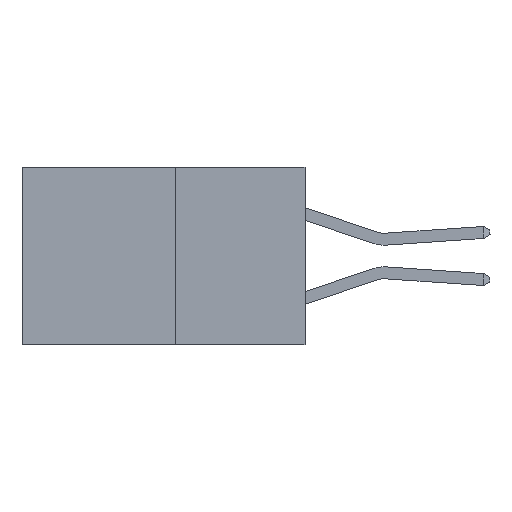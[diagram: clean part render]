
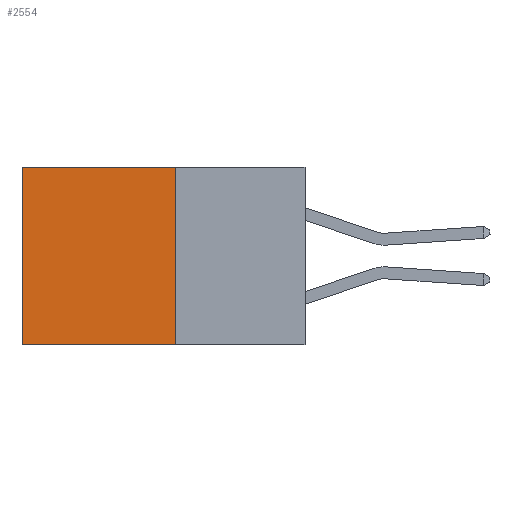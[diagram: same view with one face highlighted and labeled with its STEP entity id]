
A CAD part, left-side view. The second image highlights one B-rep face of the part: STEP entity #2554.
In plain terms, the highlighted planar face has unit normal (-1, 0, 0).
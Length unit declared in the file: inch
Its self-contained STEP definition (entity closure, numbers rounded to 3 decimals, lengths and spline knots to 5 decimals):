
#334 = ORIENTED_EDGE ( 'NONE', *, *, #688, .F. ) ;
#534 = AXIS2_PLACEMENT_3D ( 'NONE', #11192, #17111, #16595 ) ;
#688 = EDGE_CURVE ( 'NONE', #1256, #17459, #8803, .T. ) ;
#799 = ORIENTED_EDGE ( 'NONE', *, *, #17157, .F. ) ;
#933 = DIRECTION ( 'NONE',  ( 0., 1., 0. ) ) ;
#1256 = VERTEX_POINT ( 'NONE', #10063 ) ;
#1376 = EDGE_CURVE ( 'NONE', #4026, #14913, #4610, .T. ) ;
#1718 = ORIENTED_EDGE ( 'NONE', *, *, #1376, .T. ) ;
#2058 = FACE_OUTER_BOUND ( 'NONE', #18214, .T. ) ;
#2374 = CARTESIAN_POINT ( 'NONE',  ( 0.277, 0.59, -0.37 ) ) ;
#2554 = ADVANCED_FACE ( 'NONE', ( #2058 ), #17402, .F. ) ;
#2951 = LINE ( 'NONE', #19134, #11455 ) ;
#4026 = VERTEX_POINT ( 'NONE', #19067 ) ;
#4610 = LINE ( 'NONE', #9505, #8307 ) ;
#4878 = CARTESIAN_POINT ( 'NONE',  ( 0.277, 0.27, -0.37 ) ) ;
#4965 = DIRECTION ( 'NONE',  ( 0., 0., -1. ) ) ;
#6169 = VECTOR ( 'NONE', #14476, 39.37008 ) ;
#6694 = ORIENTED_EDGE ( 'NONE', *, *, #9288, .T. ) ;
#7139 = LINE ( 'NONE', #15082, #6169 ) ;
#8074 = DIRECTION ( 'NONE',  ( 0., 1., 0. ) ) ;
#8307 = VECTOR ( 'NONE', #8074, 39.37008 ) ;
#8803 = LINE ( 'NONE', #4878, #16714 ) ;
#9288 = EDGE_CURVE ( 'NONE', #14913, #17459, #7139, .T. ) ;
#9505 = CARTESIAN_POINT ( 'NONE',  ( 0.277, 0.27, 0. ) ) ;
#10063 = CARTESIAN_POINT ( 'NONE',  ( 0.277, 0.27, -0.37 ) ) ;
#11192 = CARTESIAN_POINT ( 'NONE',  ( 0.277, 0.27, -0.37 ) ) ;
#11455 = VECTOR ( 'NONE', #4965, 39.37008 ) ;
#14476 = DIRECTION ( 'NONE',  ( 0., 0., -1. ) ) ;
#14727 = CARTESIAN_POINT ( 'NONE',  ( 0.277, 0.59, 0. ) ) ;
#14913 = VERTEX_POINT ( 'NONE', #14727 ) ;
#15082 = CARTESIAN_POINT ( 'NONE',  ( 0.277, 0.59, -0.37 ) ) ;
#16595 = DIRECTION ( 'NONE',  ( 0., 0., -1. ) ) ;
#16714 = VECTOR ( 'NONE', #933, 39.37008 ) ;
#17111 = DIRECTION ( 'NONE',  ( 1., 0., 0. ) ) ;
#17157 = EDGE_CURVE ( 'NONE', #4026, #1256, #2951, .T. ) ;
#17402 = PLANE ( 'NONE',  #534 ) ;
#17459 = VERTEX_POINT ( 'NONE', #2374 ) ;
#18214 = EDGE_LOOP ( 'NONE', ( #6694, #334, #799, #1718 ) ) ;
#19067 = CARTESIAN_POINT ( 'NONE',  ( 0.277, 0.27, 0. ) ) ;
#19134 = CARTESIAN_POINT ( 'NONE',  ( 0.277, 0.27, -0.37 ) ) ;
